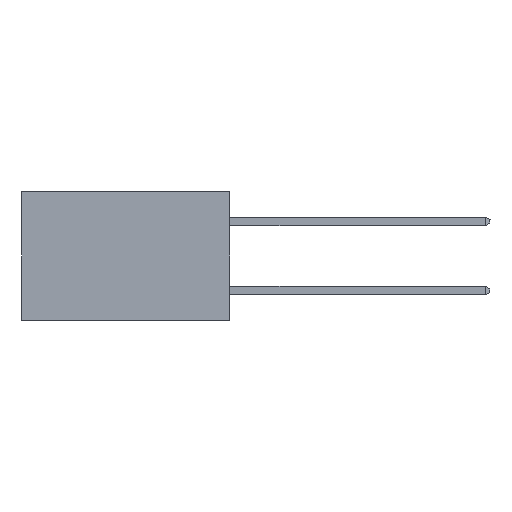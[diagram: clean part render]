
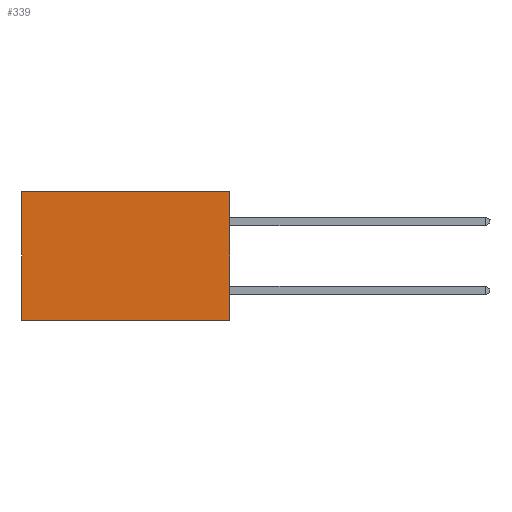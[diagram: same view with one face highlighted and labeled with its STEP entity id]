
A CAD part, left-side view. The second image highlights one B-rep face of the part: STEP entity #339.
In plain terms, the highlighted planar face has unit normal (-1, 0, 0).
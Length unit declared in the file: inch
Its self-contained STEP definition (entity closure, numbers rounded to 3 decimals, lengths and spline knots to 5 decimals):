
#28 = CARTESIAN_POINT ( 'NONE',  ( 0.298, 0., 0. ) ) ;
#48 = CARTESIAN_POINT ( 'NONE',  ( 0.298, 0., 0. ) ) ;
#165 = VERTEX_POINT ( 'NONE', #48 ) ;
#339 = ADVANCED_FACE ( 'NONE', ( #10299 ), #7701, .F. ) ;
#1477 = EDGE_CURVE ( 'NONE', #15187, #17685, #7555, .T. ) ;
#3278 = EDGE_CURVE ( 'NONE', #165, #17672, #3638, .T. ) ;
#3638 = LINE ( 'NONE', #28, #10558 ) ;
#4213 = ORIENTED_EDGE ( 'NONE', *, *, #10363, .T. ) ;
#4582 = CARTESIAN_POINT ( 'NONE',  ( 0.298, 0., 0. ) ) ;
#5516 = VECTOR ( 'NONE', #11469, 39.37008 ) ;
#5904 = AXIS2_PLACEMENT_3D ( 'NONE', #15924, #14496, #14587 ) ;
#7555 = LINE ( 'NONE', #16002, #11673 ) ;
#7701 = PLANE ( 'NONE',  #5904 ) ;
#8773 = CARTESIAN_POINT ( 'NONE',  ( 0.298, 0.6, 0. ) ) ;
#8914 = DIRECTION ( 'NONE',  ( 0., 1., 0. ) ) ;
#9186 = LINE ( 'NONE', #4582, #5516 ) ;
#9758 = DIRECTION ( 'NONE',  ( 0., 0., -1. ) ) ;
#10067 = CARTESIAN_POINT ( 'NONE',  ( 0.298, 0., -0.37 ) ) ;
#10298 = DIRECTION ( 'NONE',  ( 0., 0., -1. ) ) ;
#10299 = FACE_OUTER_BOUND ( 'NONE', #14488, .T. ) ;
#10363 = EDGE_CURVE ( 'NONE', #165, #15187, #9186, .T. ) ;
#10558 = VECTOR ( 'NONE', #9758, 39.37008 ) ;
#11325 = CARTESIAN_POINT ( 'NONE',  ( 0.298, 0., -0.37 ) ) ;
#11463 = LINE ( 'NONE', #10067, #16428 ) ;
#11469 = DIRECTION ( 'NONE',  ( 0., 1., 0. ) ) ;
#11673 = VECTOR ( 'NONE', #10298, 39.37008 ) ;
#12416 = CARTESIAN_POINT ( 'NONE',  ( 0.298, 0.6, -0.37 ) ) ;
#14199 = ORIENTED_EDGE ( 'NONE', *, *, #3278, .F. ) ;
#14488 = EDGE_LOOP ( 'NONE', ( #15776, #16337, #14199, #4213 ) ) ;
#14496 = DIRECTION ( 'NONE',  ( 1., 0., 0. ) ) ;
#14587 = DIRECTION ( 'NONE',  ( 0., 0., -1. ) ) ;
#14696 = EDGE_CURVE ( 'NONE', #17672, #17685, #11463, .T. ) ;
#15187 = VERTEX_POINT ( 'NONE', #8773 ) ;
#15776 = ORIENTED_EDGE ( 'NONE', *, *, #1477, .T. ) ;
#15924 = CARTESIAN_POINT ( 'NONE',  ( 0.298, 0., 0. ) ) ;
#16002 = CARTESIAN_POINT ( 'NONE',  ( 0.298, 0.6, 0. ) ) ;
#16337 = ORIENTED_EDGE ( 'NONE', *, *, #14696, .F. ) ;
#16428 = VECTOR ( 'NONE', #8914, 39.37008 ) ;
#17672 = VERTEX_POINT ( 'NONE', #11325 ) ;
#17685 = VERTEX_POINT ( 'NONE', #12416 ) ;
